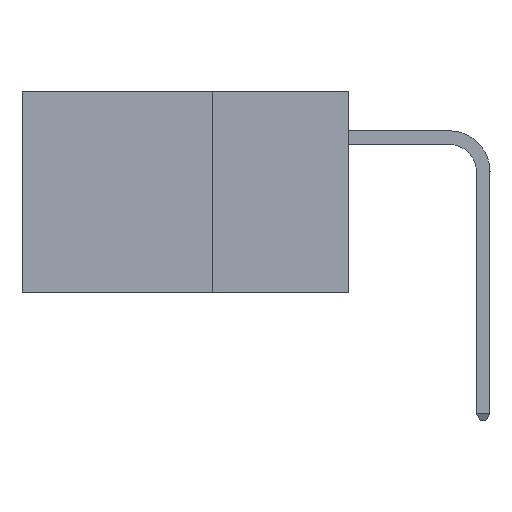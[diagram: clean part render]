
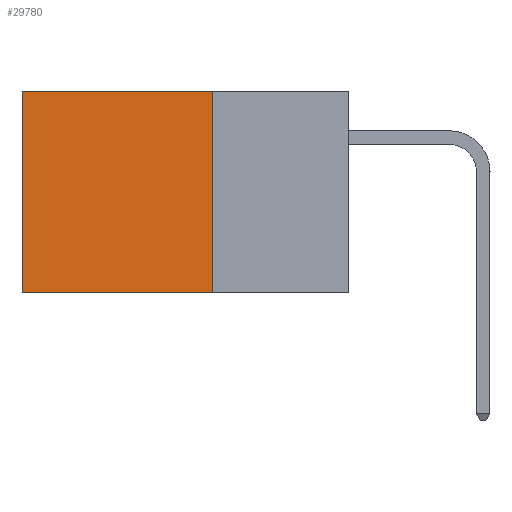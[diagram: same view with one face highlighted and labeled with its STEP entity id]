
A CAD part, left-side view. The second image highlights one B-rep face of the part: STEP entity #29780.
In plain terms, the highlighted planar face has unit normal (-1, 0, 0).
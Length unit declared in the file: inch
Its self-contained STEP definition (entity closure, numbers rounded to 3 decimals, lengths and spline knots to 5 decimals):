
#945 = CARTESIAN_POINT ( 'NONE',  ( 0.2875, 0.6, 0. ) ) ;
#1256 = EDGE_LOOP ( 'NONE', ( #30909, #6886, #22678, #1371 ) ) ;
#1371 = ORIENTED_EDGE ( 'NONE', *, *, #34146, .T. ) ;
#1489 = VECTOR ( 'NONE', #32364, 39.37008 ) ;
#4353 = CARTESIAN_POINT ( 'NONE',  ( 0.2875, 0.25, -0.37 ) ) ;
#4399 = VERTEX_POINT ( 'NONE', #30871 ) ;
#4535 = LINE ( 'NONE', #24094, #18214 ) ;
#4660 = CARTESIAN_POINT ( 'NONE',  ( 0.2875, 0.25, 0. ) ) ;
#5766 = VERTEX_POINT ( 'NONE', #4353 ) ;
#6886 = ORIENTED_EDGE ( 'NONE', *, *, #29218, .F. ) ;
#7302 = PLANE ( 'NONE',  #19892 ) ;
#7418 = DIRECTION ( 'NONE',  ( 0., 0., -1. ) ) ;
#7484 = EDGE_CURVE ( 'NONE', #13311, #14186, #20844, .T. ) ;
#7487 = VECTOR ( 'NONE', #34976, 39.37008 ) ;
#9861 = CARTESIAN_POINT ( 'NONE',  ( 0.2875, 0.6, 0. ) ) ;
#10442 = CARTESIAN_POINT ( 'NONE',  ( 0.2875, 0.25, 0. ) ) ;
#13140 = CARTESIAN_POINT ( 'NONE',  ( 0.2875, 0.25, 0. ) ) ;
#13311 = VERTEX_POINT ( 'NONE', #9861 ) ;
#13500 = VECTOR ( 'NONE', #14598, 39.37008 ) ;
#13975 = CARTESIAN_POINT ( 'NONE',  ( 0.2875, 0.6, -0.37 ) ) ;
#14186 = VERTEX_POINT ( 'NONE', #13975 ) ;
#14598 = DIRECTION ( 'NONE',  ( 0., 0., -1. ) ) ;
#15554 = LINE ( 'NONE', #13140, #7487 ) ;
#18214 = VECTOR ( 'NONE', #29610, 39.37008 ) ;
#19892 = AXIS2_PLACEMENT_3D ( 'NONE', #4660, #23818, #7418 ) ;
#20844 = LINE ( 'NONE', #945, #13500 ) ;
#22678 = ORIENTED_EDGE ( 'NONE', *, *, #34731, .F. ) ;
#23405 = LINE ( 'NONE', #10442, #1489 ) ;
#23818 = DIRECTION ( 'NONE',  ( 1., 0., 0. ) ) ;
#24094 = CARTESIAN_POINT ( 'NONE',  ( 0.2875, 0.25, -0.37 ) ) ;
#29218 = EDGE_CURVE ( 'NONE', #5766, #14186, #4535, .T. ) ;
#29610 = DIRECTION ( 'NONE',  ( 0., 1., 0. ) ) ;
#29780 = ADVANCED_FACE ( 'NONE', ( #33976 ), #7302, .F. ) ;
#30871 = CARTESIAN_POINT ( 'NONE',  ( 0.2875, 0.25, 0. ) ) ;
#30909 = ORIENTED_EDGE ( 'NONE', *, *, #7484, .T. ) ;
#32364 = DIRECTION ( 'NONE',  ( 0., 1., 0. ) ) ;
#33976 = FACE_OUTER_BOUND ( 'NONE', #1256, .T. ) ;
#34146 = EDGE_CURVE ( 'NONE', #4399, #13311, #23405, .T. ) ;
#34731 = EDGE_CURVE ( 'NONE', #4399, #5766, #15554, .T. ) ;
#34976 = DIRECTION ( 'NONE',  ( 0., 0., -1. ) ) ;
